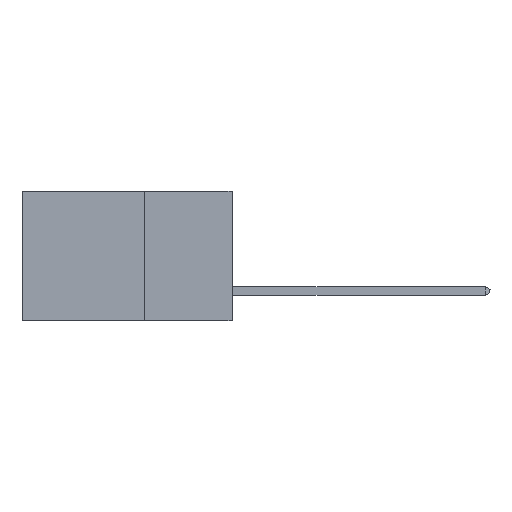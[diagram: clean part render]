
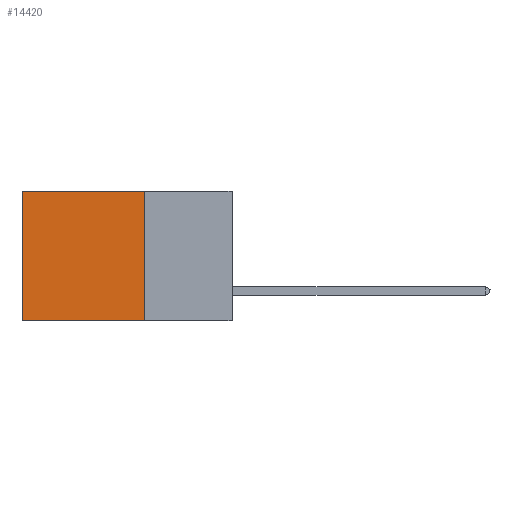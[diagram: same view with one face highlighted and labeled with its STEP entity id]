
A CAD part, left-side view. The second image highlights one B-rep face of the part: STEP entity #14420.
In plain terms, the highlighted planar face has unit normal (-1, 0, 0).
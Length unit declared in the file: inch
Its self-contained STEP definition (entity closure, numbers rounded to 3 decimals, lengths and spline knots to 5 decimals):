
#104 = CARTESIAN_POINT ( 'NONE',  ( 0.2875, 0.25, 0. ) ) ;
#1897 = VERTEX_POINT ( 'NONE', #3355 ) ;
#2524 = CARTESIAN_POINT ( 'NONE',  ( 0.2875, 0.6, -0.37 ) ) ;
#2677 = DIRECTION ( 'NONE',  ( 0., 0., -1. ) ) ;
#2698 = EDGE_CURVE ( 'NONE', #5589, #5944, #11006, .T. ) ;
#3059 = DIRECTION ( 'NONE',  ( 0., 1., 0. ) ) ;
#3355 = CARTESIAN_POINT ( 'NONE',  ( 0.2875, 0.25, 0. ) ) ;
#3710 = CARTESIAN_POINT ( 'NONE',  ( 0.2875, 0.6, 0. ) ) ;
#4650 = CARTESIAN_POINT ( 'NONE',  ( 0.2875, 0.6, 0. ) ) ;
#4670 = VECTOR ( 'NONE', #3059, 39.37008 ) ;
#5221 = VERTEX_POINT ( 'NONE', #8037 ) ;
#5589 = VERTEX_POINT ( 'NONE', #4650 ) ;
#5778 = ORIENTED_EDGE ( 'NONE', *, *, #19604, .F. ) ;
#5944 = VERTEX_POINT ( 'NONE', #2524 ) ;
#6022 = EDGE_LOOP ( 'NONE', ( #7141, #16734, #5778, #9823 ) ) ;
#7141 = ORIENTED_EDGE ( 'NONE', *, *, #2698, .T. ) ;
#7167 = DIRECTION ( 'NONE',  ( 0., 0., -1. ) ) ;
#8037 = CARTESIAN_POINT ( 'NONE',  ( 0.2875, 0.25, -0.37 ) ) ;
#8664 = VECTOR ( 'NONE', #2677, 39.37008 ) ;
#8694 = AXIS2_PLACEMENT_3D ( 'NONE', #13339, #13514, #7167 ) ;
#8777 = PLANE ( 'NONE',  #8694 ) ;
#9605 = LINE ( 'NONE', #10295, #8664 ) ;
#9823 = ORIENTED_EDGE ( 'NONE', *, *, #11153, .T. ) ;
#10295 = CARTESIAN_POINT ( 'NONE',  ( 0.2875, 0.25, 0. ) ) ;
#11006 = LINE ( 'NONE', #3710, #18027 ) ;
#11153 = EDGE_CURVE ( 'NONE', #1897, #5589, #17015, .T. ) ;
#11533 = EDGE_CURVE ( 'NONE', #5221, #5944, #13173, .T. ) ;
#12146 = DIRECTION ( 'NONE',  ( 0., 1., 0. ) ) ;
#13173 = LINE ( 'NONE', #13961, #18874 ) ;
#13339 = CARTESIAN_POINT ( 'NONE',  ( 0.2875, 0.25, 0. ) ) ;
#13514 = DIRECTION ( 'NONE',  ( 1., 0., 0. ) ) ;
#13961 = CARTESIAN_POINT ( 'NONE',  ( 0.2875, 0.25, -0.37 ) ) ;
#14420 = ADVANCED_FACE ( 'NONE', ( #15618 ), #8777, .F. ) ;
#15618 = FACE_OUTER_BOUND ( 'NONE', #6022, .T. ) ;
#16119 = DIRECTION ( 'NONE',  ( 0., 0., -1. ) ) ;
#16734 = ORIENTED_EDGE ( 'NONE', *, *, #11533, .F. ) ;
#17015 = LINE ( 'NONE', #104, #4670 ) ;
#18027 = VECTOR ( 'NONE', #16119, 39.37008 ) ;
#18874 = VECTOR ( 'NONE', #12146, 39.37008 ) ;
#19604 = EDGE_CURVE ( 'NONE', #1897, #5221, #9605, .T. ) ;
